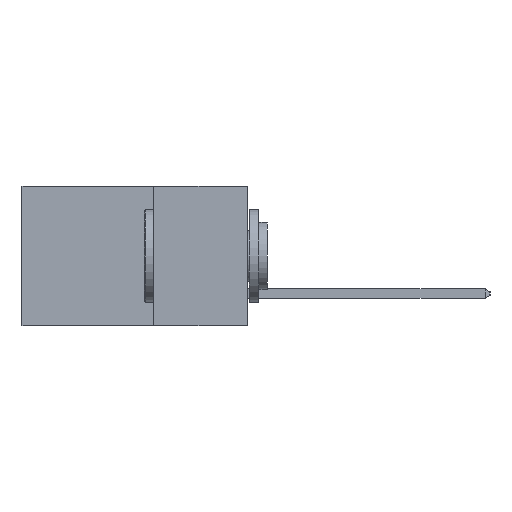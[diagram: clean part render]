
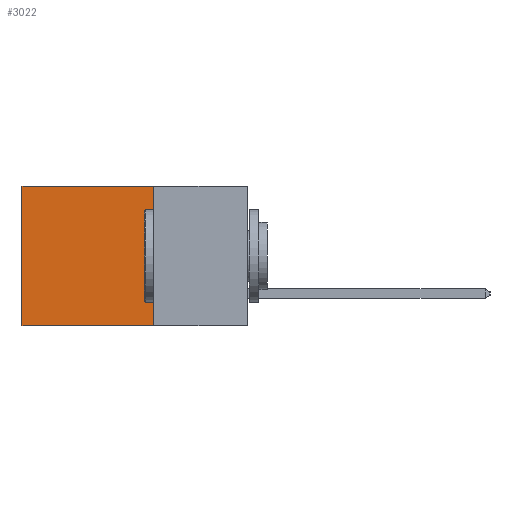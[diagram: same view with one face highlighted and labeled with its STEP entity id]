
A CAD part, left-side view. The second image highlights one B-rep face of the part: STEP entity #3022.
In plain terms, the highlighted planar face has unit normal (-1, 0, 0).
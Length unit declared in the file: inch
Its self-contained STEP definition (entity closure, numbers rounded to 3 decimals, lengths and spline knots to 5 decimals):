
#189 = FACE_OUTER_BOUND ( 'NONE', #8976, .T. ) ;
#190 = EDGE_CURVE ( 'NONE', #14089, #4659, #18922, .T. ) ;
#1575 = CARTESIAN_POINT ( 'NONE',  ( 0.298, 0.25, 0. ) ) ;
#1875 = EDGE_CURVE ( 'NONE', #6295, #9962, #8558, .T. ) ;
#2878 = VECTOR ( 'NONE', #6340, 39.37008 ) ;
#3022 = ADVANCED_FACE ( 'NONE', ( #189 ), #4772, .F. ) ;
#3232 = LINE ( 'NONE', #8519, #18660 ) ;
#4053 = CARTESIAN_POINT ( 'NONE',  ( 0.298, 0.6, -0.37 ) ) ;
#4388 = VECTOR ( 'NONE', #9052, 39.37008 ) ;
#4659 = VERTEX_POINT ( 'NONE', #23901 ) ;
#4772 = PLANE ( 'NONE',  #17339 ) ;
#6253 = EDGE_CURVE ( 'NONE', #14089, #6295, #14390, .T. ) ;
#6295 = VERTEX_POINT ( 'NONE', #10706 ) ;
#6340 = DIRECTION ( 'NONE',  ( 0., 0., -1. ) ) ;
#8519 = CARTESIAN_POINT ( 'NONE',  ( 0.298, 0.25, -0.37 ) ) ;
#8558 = LINE ( 'NONE', #9186, #4388 ) ;
#8743 = ORIENTED_EDGE ( 'NONE', *, *, #22107, .F. ) ;
#8976 = EDGE_LOOP ( 'NONE', ( #18910, #8743, #19624, #12621 ) ) ;
#9052 = DIRECTION ( 'NONE',  ( 0., 0., -1. ) ) ;
#9186 = CARTESIAN_POINT ( 'NONE',  ( 0.298, 0.6, 0. ) ) ;
#9626 = VECTOR ( 'NONE', #11233, 39.37008 ) ;
#9962 = VERTEX_POINT ( 'NONE', #4053 ) ;
#10706 = CARTESIAN_POINT ( 'NONE',  ( 0.298, 0.6, 0. ) ) ;
#11203 = CARTESIAN_POINT ( 'NONE',  ( 0.298, 0.25, 0. ) ) ;
#11233 = DIRECTION ( 'NONE',  ( 0., 1., 0. ) ) ;
#12621 = ORIENTED_EDGE ( 'NONE', *, *, #6253, .T. ) ;
#14089 = VERTEX_POINT ( 'NONE', #15464 ) ;
#14390 = LINE ( 'NONE', #11203, #9626 ) ;
#15464 = CARTESIAN_POINT ( 'NONE',  ( 0.298, 0.25, 0. ) ) ;
#17339 = AXIS2_PLACEMENT_3D ( 'NONE', #18378, #18458, #18552 ) ;
#18378 = CARTESIAN_POINT ( 'NONE',  ( 0.298, 0.25, 0. ) ) ;
#18458 = DIRECTION ( 'NONE',  ( 1., 0., 0. ) ) ;
#18552 = DIRECTION ( 'NONE',  ( 0., 0., -1. ) ) ;
#18660 = VECTOR ( 'NONE', #24274, 39.37008 ) ;
#18910 = ORIENTED_EDGE ( 'NONE', *, *, #1875, .T. ) ;
#18922 = LINE ( 'NONE', #1575, #2878 ) ;
#19624 = ORIENTED_EDGE ( 'NONE', *, *, #190, .F. ) ;
#22107 = EDGE_CURVE ( 'NONE', #4659, #9962, #3232, .T. ) ;
#23901 = CARTESIAN_POINT ( 'NONE',  ( 0.298, 0.25, -0.37 ) ) ;
#24274 = DIRECTION ( 'NONE',  ( 0., 1., 0. ) ) ;
